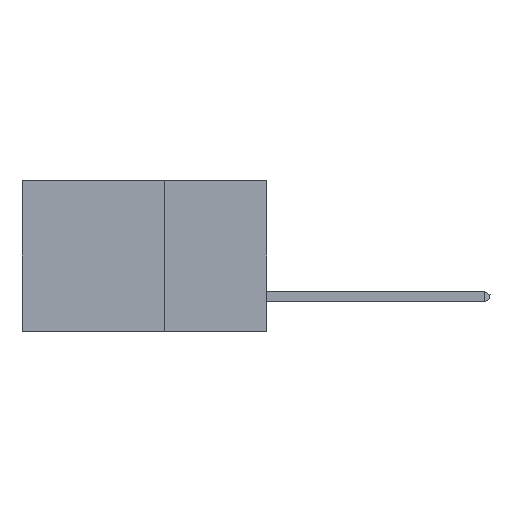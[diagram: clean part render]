
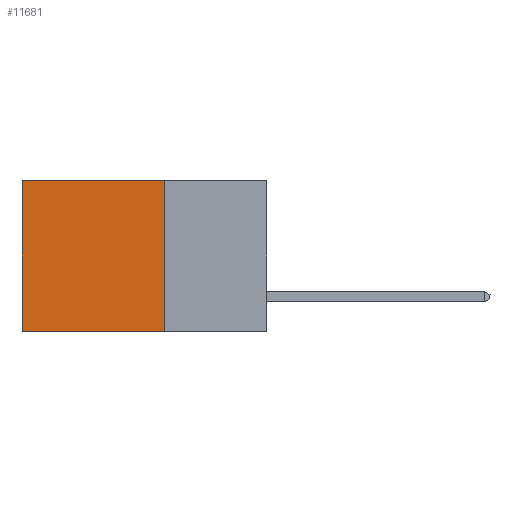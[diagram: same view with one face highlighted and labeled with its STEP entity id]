
A CAD part, left-side view. The second image highlights one B-rep face of the part: STEP entity #11681.
In plain terms, the highlighted planar face has unit normal (-1, 0, 0).
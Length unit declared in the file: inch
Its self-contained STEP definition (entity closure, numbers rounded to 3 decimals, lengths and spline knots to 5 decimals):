
#211 = CARTESIAN_POINT ( 'NONE',  ( 0.2875, 0.6, -0.37 ) ) ;
#363 = EDGE_LOOP ( 'NONE', ( #2559, #1125, #999, #8668 ) ) ;
#999 = ORIENTED_EDGE ( 'NONE', *, *, #11832, .F. ) ;
#1047 = DIRECTION ( 'NONE',  ( 0., 1., 0. ) ) ;
#1125 = ORIENTED_EDGE ( 'NONE', *, *, #4972, .F. ) ;
#1507 = VECTOR ( 'NONE', #1047, 39.37008 ) ;
#1910 = VECTOR ( 'NONE', #2564, 39.37008 ) ;
#2088 = AXIS2_PLACEMENT_3D ( 'NONE', #11671, #13823, #11609 ) ;
#2559 = ORIENTED_EDGE ( 'NONE', *, *, #10403, .T. ) ;
#2564 = DIRECTION ( 'NONE',  ( 0., 1., 0. ) ) ;
#2669 = CARTESIAN_POINT ( 'NONE',  ( 0.2875, 0.6, 0. ) ) ;
#3769 = CARTESIAN_POINT ( 'NONE',  ( 0.2875, 0.25, -0.37 ) ) ;
#4071 = LINE ( 'NONE', #10577, #5429 ) ;
#4152 = DIRECTION ( 'NONE',  ( 0., 0., -1. ) ) ;
#4402 = CARTESIAN_POINT ( 'NONE',  ( 0.2875, 0.25, 0. ) ) ;
#4633 = CARTESIAN_POINT ( 'NONE',  ( 0.2875, 0.25, -0.37 ) ) ;
#4972 = EDGE_CURVE ( 'NONE', #8292, #7907, #13443, .T. ) ;
#5137 = DIRECTION ( 'NONE',  ( 0., 0., -1. ) ) ;
#5429 = VECTOR ( 'NONE', #5137, 39.37008 ) ;
#7094 = PLANE ( 'NONE',  #2088 ) ;
#7609 = VERTEX_POINT ( 'NONE', #2669 ) ;
#7907 = VERTEX_POINT ( 'NONE', #211 ) ;
#8292 = VERTEX_POINT ( 'NONE', #3769 ) ;
#8668 = ORIENTED_EDGE ( 'NONE', *, *, #9363, .T. ) ;
#9363 = EDGE_CURVE ( 'NONE', #11111, #7609, #9631, .T. ) ;
#9631 = LINE ( 'NONE', #4402, #1507 ) ;
#10119 = CARTESIAN_POINT ( 'NONE',  ( 0.2875, 0.25, 0. ) ) ;
#10403 = EDGE_CURVE ( 'NONE', #7609, #7907, #4071, .T. ) ;
#10577 = CARTESIAN_POINT ( 'NONE',  ( 0.2875, 0.6, 0. ) ) ;
#10600 = FACE_OUTER_BOUND ( 'NONE', #363, .T. ) ;
#11111 = VERTEX_POINT ( 'NONE', #10119 ) ;
#11245 = VECTOR ( 'NONE', #4152, 39.37008 ) ;
#11609 = DIRECTION ( 'NONE',  ( 0., 0., -1. ) ) ;
#11671 = CARTESIAN_POINT ( 'NONE',  ( 0.2875, 0.25, 0. ) ) ;
#11681 = ADVANCED_FACE ( 'NONE', ( #10600 ), #7094, .F. ) ;
#11832 = EDGE_CURVE ( 'NONE', #11111, #8292, #12017, .T. ) ;
#12017 = LINE ( 'NONE', #13086, #11245 ) ;
#13086 = CARTESIAN_POINT ( 'NONE',  ( 0.2875, 0.25, 0. ) ) ;
#13443 = LINE ( 'NONE', #4633, #1910 ) ;
#13823 = DIRECTION ( 'NONE',  ( 1., 0., 0. ) ) ;
